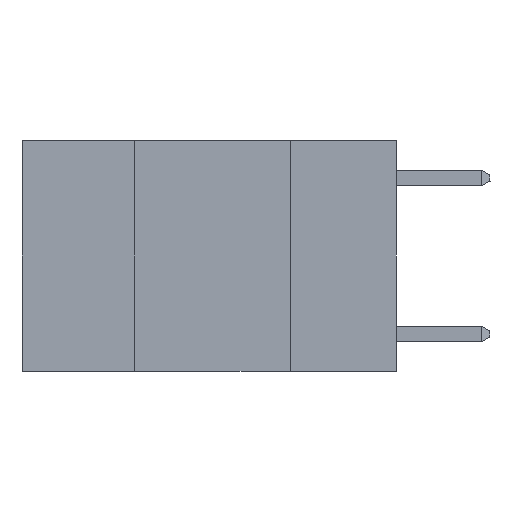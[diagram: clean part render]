
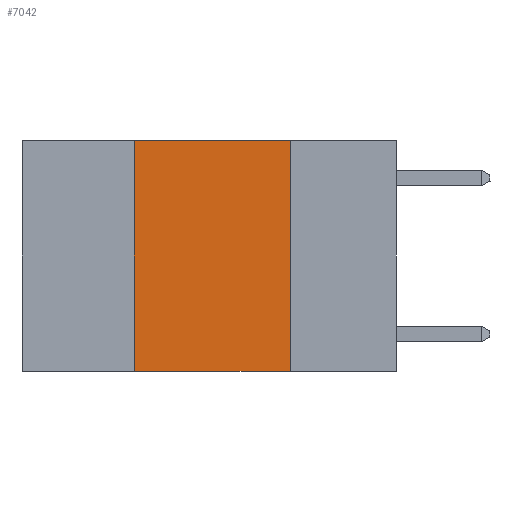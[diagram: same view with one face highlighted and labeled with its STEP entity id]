
A CAD part, left-side view. The second image highlights one B-rep face of the part: STEP entity #7042.
In plain terms, the highlighted planar face has unit normal (-1, 0, 0).
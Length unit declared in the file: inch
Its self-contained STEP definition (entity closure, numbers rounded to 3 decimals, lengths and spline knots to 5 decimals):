
#3 = CARTESIAN_POINT ( 'NONE',  ( 0., 0.6, -0.37 ) ) ;
#397 = DIRECTION ( 'NONE',  ( 0., 0., -1. ) ) ;
#467 = CARTESIAN_POINT ( 'NONE',  ( 0., 0.42, 0. ) ) ;
#508 = ORIENTED_EDGE ( 'NONE', *, *, #1668, .F. ) ;
#852 = LINE ( 'NONE', #467, #4521 ) ;
#1015 = ORIENTED_EDGE ( 'NONE', *, *, #4555, .T. ) ;
#1462 = VERTEX_POINT ( 'NONE', #2685 ) ;
#1668 = EDGE_CURVE ( 'NONE', #4956, #1462, #852, .T. ) ;
#2144 = ORIENTED_EDGE ( 'NONE', *, *, #3043, .F. ) ;
#2273 = VECTOR ( 'NONE', #6409, 39.37008 ) ;
#2527 = LINE ( 'NONE', #5727, #2273 ) ;
#2685 = CARTESIAN_POINT ( 'NONE',  ( 0., 0.42, 0. ) ) ;
#2768 = CARTESIAN_POINT ( 'NONE',  ( 0., 0.42, -0.37 ) ) ;
#3043 = EDGE_CURVE ( 'NONE', #1462, #8022, #7387, .T. ) ;
#3281 = DIRECTION ( 'NONE',  ( 0., 0., 1. ) ) ;
#3733 = ORIENTED_EDGE ( 'NONE', *, *, #4491, .F. ) ;
#3903 = VERTEX_POINT ( 'NONE', #7795 ) ;
#4355 = DIRECTION ( 'NONE',  ( 0., -1., 0. ) ) ;
#4491 = EDGE_CURVE ( 'NONE', #8022, #3903, #2527, .T. ) ;
#4521 = VECTOR ( 'NONE', #3281, 39.37008 ) ;
#4555 = EDGE_CURVE ( 'NONE', #4956, #3903, #8922, .T. ) ;
#4777 = DIRECTION ( 'NONE',  ( 1., 0., 0. ) ) ;
#4956 = VERTEX_POINT ( 'NONE', #2768 ) ;
#4995 = CARTESIAN_POINT ( 'NONE',  ( 0., 0.6, 0. ) ) ;
#5022 = CARTESIAN_POINT ( 'NONE',  ( 0., 0.17, 0. ) ) ;
#5319 = VECTOR ( 'NONE', #7099, 39.37008 ) ;
#5642 = VECTOR ( 'NONE', #4355, 39.37008 ) ;
#5727 = CARTESIAN_POINT ( 'NONE',  ( 0., 0.17, 0. ) ) ;
#6409 = DIRECTION ( 'NONE',  ( 0., 0., -1. ) ) ;
#6430 = FACE_OUTER_BOUND ( 'NONE', #8419, .T. ) ;
#7042 = ADVANCED_FACE ( 'NONE', ( #6430 ), #8645, .F. ) ;
#7099 = DIRECTION ( 'NONE',  ( 0., -1., 0. ) ) ;
#7387 = LINE ( 'NONE', #4995, #5642 ) ;
#7402 = AXIS2_PLACEMENT_3D ( 'NONE', #8671, #4777, #397 ) ;
#7795 = CARTESIAN_POINT ( 'NONE',  ( 0., 0.17, -0.37 ) ) ;
#8022 = VERTEX_POINT ( 'NONE', #5022 ) ;
#8419 = EDGE_LOOP ( 'NONE', ( #3733, #2144, #508, #1015 ) ) ;
#8645 = PLANE ( 'NONE',  #7402 ) ;
#8671 = CARTESIAN_POINT ( 'NONE',  ( 0., 0.6, 0. ) ) ;
#8922 = LINE ( 'NONE', #3, #5319 ) ;
